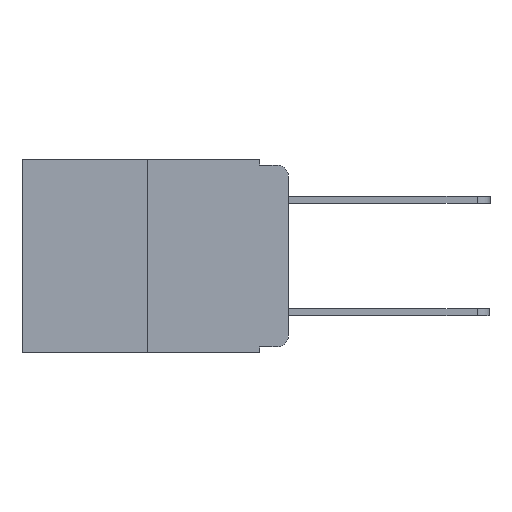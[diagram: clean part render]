
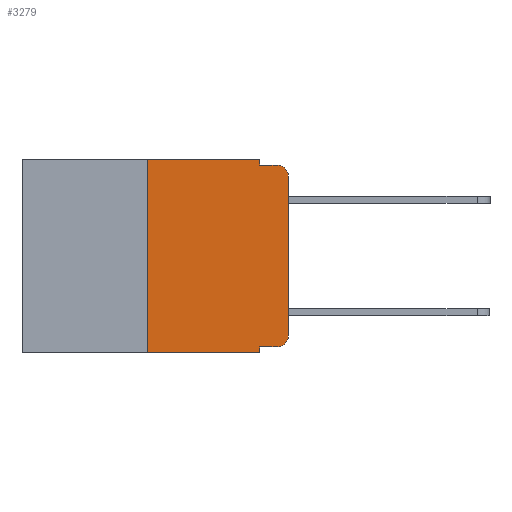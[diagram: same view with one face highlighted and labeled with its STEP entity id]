
A CAD part, left-side view. The second image highlights one B-rep face of the part: STEP entity #3279.
In plain terms, the highlighted planar face has unit normal (-1, 0, 0).
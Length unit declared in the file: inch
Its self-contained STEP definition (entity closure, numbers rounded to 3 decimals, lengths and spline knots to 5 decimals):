
#124 = FACE_OUTER_BOUND ( 'NONE', #18292, .T. ) ;
#212 = VERTEX_POINT ( 'NONE', #11086 ) ;
#231 = ORIENTED_EDGE ( 'NONE', *, *, #18731, .F. ) ;
#712 = VERTEX_POINT ( 'NONE', #18818 ) ;
#1292 = VERTEX_POINT ( 'NONE', #14634 ) ;
#1544 = VECTOR ( 'NONE', #17563, 39.37008 ) ;
#1843 = DIRECTION ( 'NONE',  ( 0., 0., 1. ) ) ;
#2073 = ORIENTED_EDGE ( 'NONE', *, *, #8956, .T. ) ;
#2271 = LINE ( 'NONE', #3751, #6280 ) ;
#2482 = CARTESIAN_POINT ( 'NONE',  ( 0., 0.051, 0. ) ) ;
#2654 = VERTEX_POINT ( 'NONE', #8070 ) ;
#2776 = ORIENTED_EDGE ( 'NONE', *, *, #19094, .T. ) ;
#2880 = CARTESIAN_POINT ( 'NONE',  ( 0., 0.25, -0.343 ) ) ;
#2953 = ORIENTED_EDGE ( 'NONE', *, *, #6515, .T. ) ;
#2993 = EDGE_CURVE ( 'NONE', #2654, #16039, #18138, .T. ) ;
#3279 = ADVANCED_FACE ( 'NONE', ( #124 ), #4979, .F. ) ;
#3368 = DIRECTION ( 'NONE',  ( -1., 0., 0. ) ) ;
#3516 = CARTESIAN_POINT ( 'NONE',  ( 0., 0.473, 0. ) ) ;
#3751 = CARTESIAN_POINT ( 'NONE',  ( 0., 0.051, -0.333 ) ) ;
#4041 = CARTESIAN_POINT ( 'NONE',  ( 0., 0., -0.03 ) ) ;
#4270 = CARTESIAN_POINT ( 'NONE',  ( 0., 0.051, -0.333 ) ) ;
#4504 = VECTOR ( 'NONE', #5264, 39.37008 ) ;
#4588 = EDGE_CURVE ( 'NONE', #7991, #9168, #16542, .T. ) ;
#4746 = CARTESIAN_POINT ( 'NONE',  ( 0., 0.25, 0. ) ) ;
#4979 = PLANE ( 'NONE',  #18368 ) ;
#5264 = DIRECTION ( 'NONE',  ( 0., -1., 0. ) ) ;
#5335 = ORIENTED_EDGE ( 'NONE', *, *, #13730, .F. ) ;
#5851 = ORIENTED_EDGE ( 'NONE', *, *, #6416, .F. ) ;
#6033 = ORIENTED_EDGE ( 'NONE', *, *, #4588, .T. ) ;
#6280 = VECTOR ( 'NONE', #11546, 39.37008 ) ;
#6416 = EDGE_CURVE ( 'NONE', #212, #2654, #14393, .T. ) ;
#6425 = CARTESIAN_POINT ( 'NONE',  ( 0., 0., -0.313 ) ) ;
#6515 = EDGE_CURVE ( 'NONE', #712, #7991, #15520, .T. ) ;
#6517 = VECTOR ( 'NONE', #12843, 39.37008 ) ;
#7991 = VERTEX_POINT ( 'NONE', #6425 ) ;
#8070 = CARTESIAN_POINT ( 'NONE',  ( 0., 0.051, -0.01 ) ) ;
#8190 = DIRECTION ( 'NONE',  ( 0., 0., -1. ) ) ;
#8872 = EDGE_CURVE ( 'NONE', #9168, #16039, #15204, .T. ) ;
#8956 = EDGE_CURVE ( 'NONE', #12930, #1292, #10537, .T. ) ;
#9107 = ORIENTED_EDGE ( 'NONE', *, *, #12153, .F. ) ;
#9168 = VERTEX_POINT ( 'NONE', #4041 ) ;
#9599 = DIRECTION ( 'NONE',  ( -1., 0., 0. ) ) ;
#9893 = LINE ( 'NONE', #10823, #16121 ) ;
#10144 = AXIS2_PLACEMENT_3D ( 'NONE', #18083, #9599, #19468 ) ;
#10537 = LINE ( 'NONE', #18433, #6517 ) ;
#10709 = CARTESIAN_POINT ( 'NONE',  ( 0., 0.051, 0. ) ) ;
#10823 = CARTESIAN_POINT ( 'NONE',  ( 0., 0.25, 0. ) ) ;
#11086 = CARTESIAN_POINT ( 'NONE',  ( 0., 0.051, 0. ) ) ;
#11377 = AXIS2_PLACEMENT_3D ( 'NONE', #12667, #3368, #14079 ) ;
#11546 = DIRECTION ( 'NONE',  ( 0., -1., 0. ) ) ;
#11903 = DIRECTION ( 'NONE',  ( 0., 0., -1. ) ) ;
#12085 = VERTEX_POINT ( 'NONE', #4270 ) ;
#12153 = EDGE_CURVE ( 'NONE', #12085, #1292, #15329, .T. ) ;
#12627 = LINE ( 'NONE', #3516, #4504 ) ;
#12667 = CARTESIAN_POINT ( 'NONE',  ( 0., 0.02, -0.03 ) ) ;
#12843 = DIRECTION ( 'NONE',  ( 0., -1., 0. ) ) ;
#12930 = VERTEX_POINT ( 'NONE', #2880 ) ;
#13078 = CARTESIAN_POINT ( 'NONE',  ( 0., 0.02, -0.01 ) ) ;
#13286 = CARTESIAN_POINT ( 'NONE',  ( 0., 0.051, -0.01 ) ) ;
#13730 = EDGE_CURVE ( 'NONE', #19465, #212, #12627, .T. ) ;
#13967 = VECTOR ( 'NONE', #11903, 39.37008 ) ;
#14079 = DIRECTION ( 'NONE',  ( 0., 0., -1. ) ) ;
#14393 = LINE ( 'NONE', #2482, #13967 ) ;
#14634 = CARTESIAN_POINT ( 'NONE',  ( 0., 0.051, -0.343 ) ) ;
#14677 = ORIENTED_EDGE ( 'NONE', *, *, #2993, .F. ) ;
#15156 = ORIENTED_EDGE ( 'NONE', *, *, #8872, .T. ) ;
#15204 = CIRCLE ( 'NONE', #11377, 0.02 ) ;
#15329 = LINE ( 'NONE', #10709, #19046 ) ;
#15384 = CARTESIAN_POINT ( 'NONE',  ( 0., 0.473, 0. ) ) ;
#15520 = CIRCLE ( 'NONE', #10144, 0.02 ) ;
#15656 = VECTOR ( 'NONE', #1843, 39.37008 ) ;
#16039 = VERTEX_POINT ( 'NONE', #13078 ) ;
#16121 = VECTOR ( 'NONE', #17818, 39.37008 ) ;
#16542 = LINE ( 'NONE', #17017, #15656 ) ;
#16811 = DIRECTION ( 'NONE',  ( 1., 0., 0. ) ) ;
#17017 = CARTESIAN_POINT ( 'NONE',  ( 0., 0., 0. ) ) ;
#17563 = DIRECTION ( 'NONE',  ( 0., -1., 0. ) ) ;
#17767 = DIRECTION ( 'NONE',  ( 0., 0., -1. ) ) ;
#17818 = DIRECTION ( 'NONE',  ( 0., 0., 1. ) ) ;
#18083 = CARTESIAN_POINT ( 'NONE',  ( 0., 0.02, -0.313 ) ) ;
#18138 = LINE ( 'NONE', #13286, #1544 ) ;
#18292 = EDGE_LOOP ( 'NONE', ( #6033, #15156, #14677, #5851, #5335, #231, #2073, #9107, #2776, #2953 ) ) ;
#18368 = AXIS2_PLACEMENT_3D ( 'NONE', #15384, #16811, #8190 ) ;
#18433 = CARTESIAN_POINT ( 'NONE',  ( 0., 0.473, -0.343 ) ) ;
#18731 = EDGE_CURVE ( 'NONE', #12930, #19465, #9893, .T. ) ;
#18818 = CARTESIAN_POINT ( 'NONE',  ( 0., 0.02, -0.333 ) ) ;
#19046 = VECTOR ( 'NONE', #17767, 39.37008 ) ;
#19094 = EDGE_CURVE ( 'NONE', #12085, #712, #2271, .T. ) ;
#19465 = VERTEX_POINT ( 'NONE', #4746 ) ;
#19468 = DIRECTION ( 'NONE',  ( 0., 0., -1. ) ) ;
